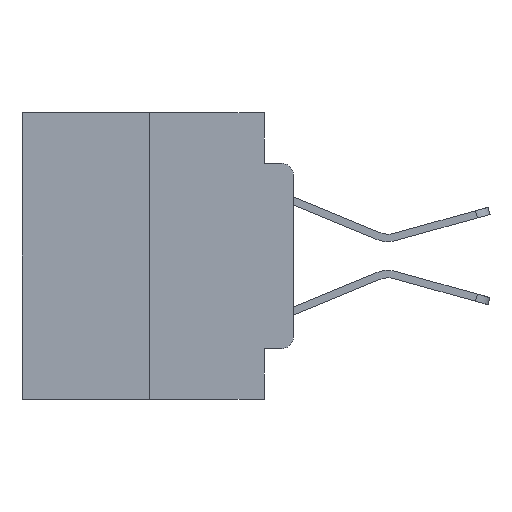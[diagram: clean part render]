
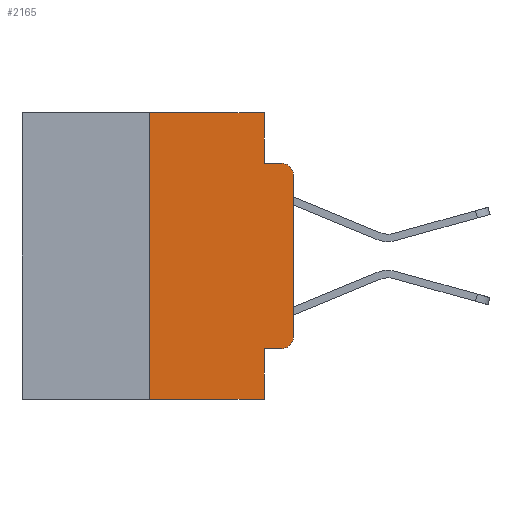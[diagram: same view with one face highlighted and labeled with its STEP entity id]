
A CAD part, left-side view. The second image highlights one B-rep face of the part: STEP entity #2165.
In plain terms, the highlighted planar face has unit normal (-1, 0, 0).
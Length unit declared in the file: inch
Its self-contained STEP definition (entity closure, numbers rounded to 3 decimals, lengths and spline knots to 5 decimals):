
#781 = CARTESIAN_POINT ( 'NONE',  ( 0., 0.02, -0.4115 ) ) ;
#860 = DIRECTION ( 'NONE',  ( 0., -1., 0. ) ) ;
#1270 = CARTESIAN_POINT ( 'NONE',  ( 0., 0.051, 0. ) ) ;
#1811 = VERTEX_POINT ( 'NONE', #21797 ) ;
#2151 = DIRECTION ( 'NONE',  ( 0., -1., 0. ) ) ;
#2153 = LINE ( 'NONE', #5714, #8378 ) ;
#2165 = ADVANCED_FACE ( 'NONE', ( #19911 ), #22305, .F. ) ;
#2229 = VERTEX_POINT ( 'NONE', #20760 ) ;
#3219 = VERTEX_POINT ( 'NONE', #13559 ) ;
#3362 = EDGE_CURVE ( 'NONE', #3219, #3919, #4918, .T. ) ;
#3886 = AXIS2_PLACEMENT_3D ( 'NONE', #24815, #22965, #25074 ) ;
#3919 = VERTEX_POINT ( 'NONE', #20189 ) ;
#4918 = LINE ( 'NONE', #24289, #20958 ) ;
#5605 = EDGE_CURVE ( 'NONE', #25099, #9269, #14280, .T. ) ;
#5689 = EDGE_CURVE ( 'NONE', #2229, #3919, #23471, .T. ) ;
#5714 = CARTESIAN_POINT ( 'NONE',  ( 0., 0., 0. ) ) ;
#5964 = EDGE_CURVE ( 'NONE', #24081, #10528, #2153, .T. ) ;
#6607 = DIRECTION ( 'NONE',  ( 0., 0., -1. ) ) ;
#7279 = CARTESIAN_POINT ( 'NONE',  ( 0., 0.473, 0. ) ) ;
#7642 = EDGE_CURVE ( 'NONE', #1811, #25099, #22345, .T. ) ;
#8378 = VECTOR ( 'NONE', #9988, 39.37008 ) ;
#9269 = VERTEX_POINT ( 'NONE', #22561 ) ;
#9988 = DIRECTION ( 'NONE',  ( 0., 0., 1. ) ) ;
#10366 = VERTEX_POINT ( 'NONE', #781 ) ;
#10403 = LINE ( 'NONE', #25827, #21256 ) ;
#10459 = ORIENTED_EDGE ( 'NONE', *, *, #10711, .F. ) ;
#10528 = VERTEX_POINT ( 'NONE', #13864 ) ;
#10711 = EDGE_CURVE ( 'NONE', #3219, #1811, #10403, .T. ) ;
#11360 = DIRECTION ( 'NONE',  ( -1., 0., 0. ) ) ;
#12100 = ORIENTED_EDGE ( 'NONE', *, *, #5689, .F. ) ;
#12525 = ORIENTED_EDGE ( 'NONE', *, *, #5605, .F. ) ;
#12592 = CARTESIAN_POINT ( 'NONE',  ( 0., 0.051, -0.4115 ) ) ;
#12948 = CARTESIAN_POINT ( 'NONE',  ( 0., 0.051, 0. ) ) ;
#13077 = DIRECTION ( 'NONE',  ( 0., 0., 1. ) ) ;
#13559 = CARTESIAN_POINT ( 'NONE',  ( 0., 0.25, -0.5 ) ) ;
#13657 = CARTESIAN_POINT ( 'NONE',  ( 0., 0.02, -0.0885 ) ) ;
#13864 = CARTESIAN_POINT ( 'NONE',  ( 0., 0., -0.1085 ) ) ;
#14280 = LINE ( 'NONE', #12948, #22476 ) ;
#14294 = EDGE_CURVE ( 'NONE', #9269, #19252, #20691, .T. ) ;
#15350 = ORIENTED_EDGE ( 'NONE', *, *, #3362, .T. ) ;
#15908 = VECTOR ( 'NONE', #19734, 39.37008 ) ;
#16443 = DIRECTION ( 'NONE',  ( 0., -1., 0. ) ) ;
#16695 = AXIS2_PLACEMENT_3D ( 'NONE', #23833, #11360, #23649 ) ;
#17405 = VECTOR ( 'NONE', #16443, 39.37008 ) ;
#17619 = CARTESIAN_POINT ( 'NONE',  ( 0., 0.051, 0. ) ) ;
#17787 = VECTOR ( 'NONE', #2151, 39.37008 ) ;
#18143 = CARTESIAN_POINT ( 'NONE',  ( 0., 0., -0.3915 ) ) ;
#18460 = DIRECTION ( 'NONE',  ( 0., 0., -1. ) ) ;
#19209 = AXIS2_PLACEMENT_3D ( 'NONE', #24437, #26522, #18460 ) ;
#19252 = VERTEX_POINT ( 'NONE', #13657 ) ;
#19734 = DIRECTION ( 'NONE',  ( 0., 0., -1. ) ) ;
#19911 = FACE_OUTER_BOUND ( 'NONE', #23704, .T. ) ;
#20189 = CARTESIAN_POINT ( 'NONE',  ( 0., 0.051, -0.5 ) ) ;
#20354 = ORIENTED_EDGE ( 'NONE', *, *, #14294, .F. ) ;
#20691 = LINE ( 'NONE', #24903, #17405 ) ;
#20760 = CARTESIAN_POINT ( 'NONE',  ( 0., 0.051, -0.4115 ) ) ;
#20810 = EDGE_CURVE ( 'NONE', #2229, #10366, #26952, .T. ) ;
#20958 = VECTOR ( 'NONE', #26383, 39.37008 ) ;
#21256 = VECTOR ( 'NONE', #13077, 39.37008 ) ;
#21795 = CIRCLE ( 'NONE', #3886, 0.02 ) ;
#21797 = CARTESIAN_POINT ( 'NONE',  ( 0., 0.25, 0. ) ) ;
#21970 = EDGE_CURVE ( 'NONE', #10366, #24081, #21795, .T. ) ;
#22004 = ORIENTED_EDGE ( 'NONE', *, *, #5964, .T. ) ;
#22017 = CIRCLE ( 'NONE', #16695, 0.02 ) ;
#22038 = VECTOR ( 'NONE', #860, 39.37008 ) ;
#22305 = PLANE ( 'NONE',  #19209 ) ;
#22341 = ORIENTED_EDGE ( 'NONE', *, *, #20810, .T. ) ;
#22345 = LINE ( 'NONE', #7279, #22038 ) ;
#22476 = VECTOR ( 'NONE', #6607, 39.37008 ) ;
#22561 = CARTESIAN_POINT ( 'NONE',  ( 0., 0.051, -0.0885 ) ) ;
#22965 = DIRECTION ( 'NONE',  ( -1., 0., 0. ) ) ;
#23471 = LINE ( 'NONE', #17619, #15908 ) ;
#23473 = ORIENTED_EDGE ( 'NONE', *, *, #24434, .T. ) ;
#23549 = ORIENTED_EDGE ( 'NONE', *, *, #21970, .T. ) ;
#23649 = DIRECTION ( 'NONE',  ( 0., 0., -1. ) ) ;
#23704 = EDGE_LOOP ( 'NONE', ( #22004, #23473, #20354, #12525, #24890, #10459, #15350, #12100, #22341, #23549 ) ) ;
#23833 = CARTESIAN_POINT ( 'NONE',  ( 0., 0.02, -0.1085 ) ) ;
#24081 = VERTEX_POINT ( 'NONE', #18143 ) ;
#24289 = CARTESIAN_POINT ( 'NONE',  ( 0., 0.473, -0.5 ) ) ;
#24434 = EDGE_CURVE ( 'NONE', #10528, #19252, #22017, .T. ) ;
#24437 = CARTESIAN_POINT ( 'NONE',  ( 0., 0.473, 0. ) ) ;
#24815 = CARTESIAN_POINT ( 'NONE',  ( 0., 0.02, -0.3915 ) ) ;
#24890 = ORIENTED_EDGE ( 'NONE', *, *, #7642, .F. ) ;
#24903 = CARTESIAN_POINT ( 'NONE',  ( 0., 0.051, -0.0885 ) ) ;
#25074 = DIRECTION ( 'NONE',  ( 0., 0., -1. ) ) ;
#25099 = VERTEX_POINT ( 'NONE', #1270 ) ;
#25827 = CARTESIAN_POINT ( 'NONE',  ( 0., 0.25, 0. ) ) ;
#26383 = DIRECTION ( 'NONE',  ( 0., -1., 0. ) ) ;
#26522 = DIRECTION ( 'NONE',  ( 1., 0., 0. ) ) ;
#26952 = LINE ( 'NONE', #12592, #17787 ) ;
